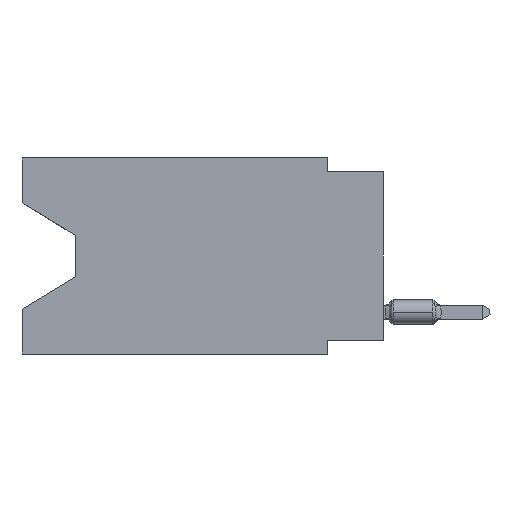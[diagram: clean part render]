
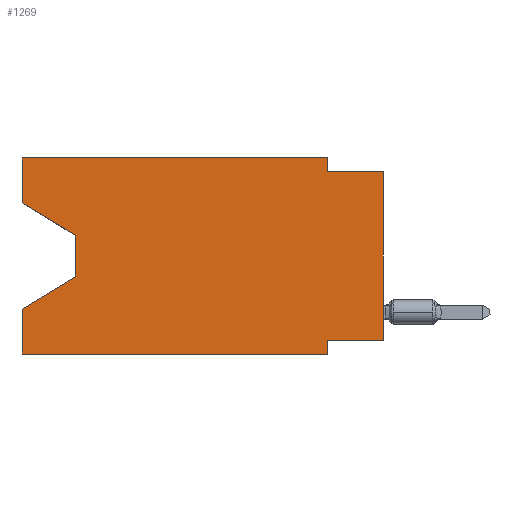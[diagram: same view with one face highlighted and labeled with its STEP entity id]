
A CAD part, left-side view. The second image highlights one B-rep face of the part: STEP entity #1269.
In plain terms, the highlighted planar face has unit normal (-1, 0, 0).
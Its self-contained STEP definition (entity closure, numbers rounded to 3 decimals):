
#131 = DIRECTION ( 'NONE',  ( 1., 0., 0. ) ) ;
#699 = CARTESIAN_POINT ( 'NONE',  ( 0., 13.97, -5.385 ) ) ;
#744 = ORIENTED_EDGE ( 'NONE', *, *, #16981, .T. ) ;
#759 = DIRECTION ( 'NONE',  ( 0., 0., 1. ) ) ;
#1167 = VECTOR ( 'NONE', #9744, 1000. ) ;
#1269 = ADVANCED_FACE ( 'NONE', ( #8100 ), #9549, .F. ) ;
#1740 = DIRECTION ( 'NONE',  ( 0., 0., 1. ) ) ;
#1804 = VERTEX_POINT ( 'NONE', #8474 ) ;
#1807 = VERTEX_POINT ( 'NONE', #4503 ) ;
#1818 = EDGE_CURVE ( 'NONE', #7966, #6936, #11371, .T. ) ;
#1822 = CARTESIAN_POINT ( 'NONE',  ( 0., 0., 0. ) ) ;
#2007 = CARTESIAN_POINT ( 'NONE',  ( 0., 2.54, -8.255 ) ) ;
#2071 = CARTESIAN_POINT ( 'NONE',  ( 0., 16.383, -8.89 ) ) ;
#2147 = VECTOR ( 'NONE', #12767, 1000. ) ;
#2647 = VERTEX_POINT ( 'NONE', #8344 ) ;
#2827 = LINE ( 'NONE', #1822, #8236 ) ;
#2847 = CARTESIAN_POINT ( 'NONE',  ( 0., 16.383, -2.038 ) ) ;
#3237 = DIRECTION ( 'NONE',  ( 0., -1., 0. ) ) ;
#3244 = EDGE_CURVE ( 'NONE', #9423, #3352, #6042, .T. ) ;
#3290 = CARTESIAN_POINT ( 'NONE',  ( 0., 0., -8.255 ) ) ;
#3352 = VERTEX_POINT ( 'NONE', #17706 ) ;
#3361 = VECTOR ( 'NONE', #14375, 1000. ) ;
#3698 = CARTESIAN_POINT ( 'NONE',  ( 0., 13.97, -3.505 ) ) ;
#3967 = CARTESIAN_POINT ( 'NONE',  ( 0., 2.54, -8.89 ) ) ;
#4125 = EDGE_CURVE ( 'NONE', #11305, #15096, #15595, .T. ) ;
#4220 = ORIENTED_EDGE ( 'NONE', *, *, #16270, .F. ) ;
#4444 = CARTESIAN_POINT ( 'NONE',  ( 0., 0., -0.635 ) ) ;
#4503 = CARTESIAN_POINT ( 'NONE',  ( 0., 0., -0.635 ) ) ;
#4729 = EDGE_CURVE ( 'NONE', #15096, #9423, #12800, .T. ) ;
#5230 = LINE ( 'NONE', #10747, #1167 ) ;
#5313 = CARTESIAN_POINT ( 'NONE',  ( 0., 2.54, 0. ) ) ;
#5505 = DIRECTION ( 'NONE',  ( 0., -1., 0. ) ) ;
#5860 = ORIENTED_EDGE ( 'NONE', *, *, #11916, .F. ) ;
#6042 = LINE ( 'NONE', #11741, #3361 ) ;
#6257 = CARTESIAN_POINT ( 'NONE',  ( 0., 16.383, 0. ) ) ;
#6268 = VERTEX_POINT ( 'NONE', #3290 ) ;
#6706 = EDGE_CURVE ( 'NONE', #2647, #1807, #11321, .T. ) ;
#6936 = VERTEX_POINT ( 'NONE', #8467 ) ;
#7944 = DIRECTION ( 'NONE',  ( 0., 0., -1. ) ) ;
#7966 = VERTEX_POINT ( 'NONE', #6257 ) ;
#8100 = FACE_OUTER_BOUND ( 'NONE', #16634, .T. ) ;
#8236 = VECTOR ( 'NONE', #1740, 1000. ) ;
#8344 = CARTESIAN_POINT ( 'NONE',  ( 0., 2.54, -0.635 ) ) ;
#8467 = CARTESIAN_POINT ( 'NONE',  ( 0., 2.54, 0. ) ) ;
#8474 = CARTESIAN_POINT ( 'NONE',  ( 0., 16.383, -8.89 ) ) ;
#8518 = ORIENTED_EDGE ( 'NONE', *, *, #1818, .F. ) ;
#8553 = DIRECTION ( 'NONE',  ( 0., 0., -1. ) ) ;
#8658 = ORIENTED_EDGE ( 'NONE', *, *, #4729, .T. ) ;
#8889 = ORIENTED_EDGE ( 'NONE', *, *, #12669, .F. ) ;
#8990 = CARTESIAN_POINT ( 'NONE',  ( 0., 16.383, -2.038 ) ) ;
#9121 = LINE ( 'NONE', #2071, #14815 ) ;
#9423 = VERTEX_POINT ( 'NONE', #699 ) ;
#9549 = PLANE ( 'NONE',  #10640 ) ;
#9744 = DIRECTION ( 'NONE',  ( 0., 0., 1. ) ) ;
#9822 = DIRECTION ( 'NONE',  ( 0., 0., -1. ) ) ;
#9823 = CARTESIAN_POINT ( 'NONE',  ( 0., 16.383, 0. ) ) ;
#9927 = DIRECTION ( 'NONE',  ( 0., 1., 0. ) ) ;
#10165 = VERTEX_POINT ( 'NONE', #2007 ) ;
#10577 = EDGE_CURVE ( 'NONE', #1804, #17357, #9121, .T. ) ;
#10640 = AXIS2_PLACEMENT_3D ( 'NONE', #9823, #131, #15336 ) ;
#10747 = CARTESIAN_POINT ( 'NONE',  ( 0., 16.383, 0. ) ) ;
#10854 = ORIENTED_EDGE ( 'NONE', *, *, #6706, .F. ) ;
#11103 = CARTESIAN_POINT ( 'NONE',  ( 0., 16.383, 0. ) ) ;
#11305 = VERTEX_POINT ( 'NONE', #2847 ) ;
#11321 = LINE ( 'NONE', #4444, #2147 ) ;
#11371 = LINE ( 'NONE', #11103, #11510 ) ;
#11466 = VECTOR ( 'NONE', #14511, 1000. ) ;
#11510 = VECTOR ( 'NONE', #5505, 1000. ) ;
#11741 = CARTESIAN_POINT ( 'NONE',  ( 0., 13.97, -5.385 ) ) ;
#11916 = EDGE_CURVE ( 'NONE', #6936, #2647, #17713, .T. ) ;
#12082 = EDGE_CURVE ( 'NONE', #11305, #7966, #5230, .T. ) ;
#12368 = ORIENTED_EDGE ( 'NONE', *, *, #15106, .F. ) ;
#12394 = CARTESIAN_POINT ( 'NONE',  ( 0., 2.54, -8.89 ) ) ;
#12426 = VECTOR ( 'NONE', #7944, 1000. ) ;
#12461 = CARTESIAN_POINT ( 'NONE',  ( 0., 0., -8.255 ) ) ;
#12558 = ORIENTED_EDGE ( 'NONE', *, *, #10577, .T. ) ;
#12669 = EDGE_CURVE ( 'NONE', #1804, #3352, #14517, .T. ) ;
#12767 = DIRECTION ( 'NONE',  ( 0., -1., 0. ) ) ;
#12800 = LINE ( 'NONE', #15527, #13708 ) ;
#12835 = VECTOR ( 'NONE', #9927, 1000. ) ;
#13153 = CARTESIAN_POINT ( 'NONE',  ( 0., 16.383, 0. ) ) ;
#13396 = VECTOR ( 'NONE', #9822, 1000. ) ;
#13565 = ORIENTED_EDGE ( 'NONE', *, *, #3244, .T. ) ;
#13708 = VECTOR ( 'NONE', #8553, 1000. ) ;
#14201 = ORIENTED_EDGE ( 'NONE', *, *, #4125, .T. ) ;
#14375 = DIRECTION ( 'NONE',  ( 0., 0.855, -0.519 ) ) ;
#14511 = DIRECTION ( 'NONE',  ( 0., -0.855, -0.519 ) ) ;
#14517 = LINE ( 'NONE', #13153, #15056 ) ;
#14815 = VECTOR ( 'NONE', #3237, 1000. ) ;
#15056 = VECTOR ( 'NONE', #759, 1000. ) ;
#15096 = VERTEX_POINT ( 'NONE', #3698 ) ;
#15106 = EDGE_CURVE ( 'NONE', #10165, #17357, #16364, .T. ) ;
#15336 = DIRECTION ( 'NONE',  ( 0., 0., -1. ) ) ;
#15527 = CARTESIAN_POINT ( 'NONE',  ( 0., 13.97, -3.505 ) ) ;
#15539 = LINE ( 'NONE', #12461, #12835 ) ;
#15595 = LINE ( 'NONE', #8990, #11466 ) ;
#15652 = ORIENTED_EDGE ( 'NONE', *, *, #12082, .F. ) ;
#16270 = EDGE_CURVE ( 'NONE', #6268, #10165, #15539, .T. ) ;
#16364 = LINE ( 'NONE', #3967, #13396 ) ;
#16634 = EDGE_LOOP ( 'NONE', ( #14201, #8658, #13565, #8889, #12558, #12368, #4220, #744, #10854, #5860, #8518, #15652 ) ) ;
#16981 = EDGE_CURVE ( 'NONE', #6268, #1807, #2827, .T. ) ;
#17357 = VERTEX_POINT ( 'NONE', #12394 ) ;
#17706 = CARTESIAN_POINT ( 'NONE',  ( 0., 16.383, -6.852 ) ) ;
#17713 = LINE ( 'NONE', #5313, #12426 ) ;
